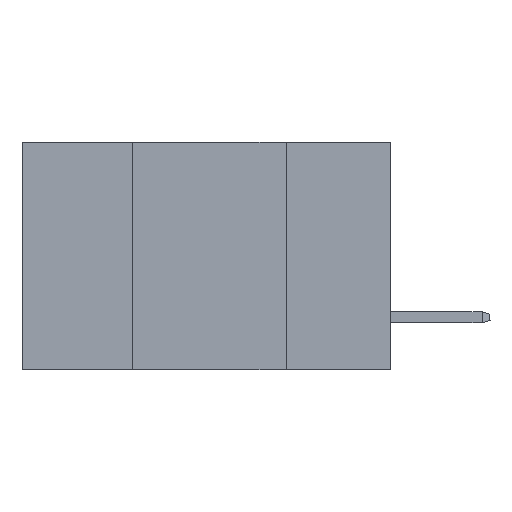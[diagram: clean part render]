
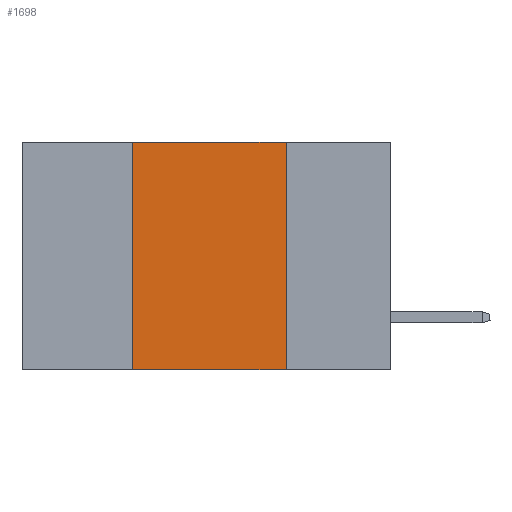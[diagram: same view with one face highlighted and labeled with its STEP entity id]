
A CAD part, left-side view. The second image highlights one B-rep face of the part: STEP entity #1698.
In plain terms, the highlighted planar face has unit normal (-1, 0, 0).
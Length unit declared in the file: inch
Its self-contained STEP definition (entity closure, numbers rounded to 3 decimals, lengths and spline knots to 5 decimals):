
#1095 = EDGE_CURVE ( 'NONE', #9346, #10973, #15724, .T. ) ;
#1698 = ADVANCED_FACE ( 'NONE', ( #9740 ), #7026, .F. ) ;
#1871 = DIRECTION ( 'NONE',  ( 1., 0., 0. ) ) ;
#2269 = DIRECTION ( 'NONE',  ( 0., -1., 0. ) ) ;
#2496 = ORIENTED_EDGE ( 'NONE', *, *, #2979, .F. ) ;
#2635 = EDGE_CURVE ( 'NONE', #7552, #4142, #11220, .T. ) ;
#2979 = EDGE_CURVE ( 'NONE', #9346, #7552, #15847, .T. ) ;
#3307 = CARTESIAN_POINT ( 'NONE',  ( 0., 0.17, 0. ) ) ;
#4142 = VERTEX_POINT ( 'NONE', #6917 ) ;
#4414 = CARTESIAN_POINT ( 'NONE',  ( 0., 0.42, 0. ) ) ;
#5377 = CARTESIAN_POINT ( 'NONE',  ( 0., 0.6, 0. ) ) ;
#5730 = CARTESIAN_POINT ( 'NONE',  ( 0., 0.42, -0.37 ) ) ;
#5921 = VECTOR ( 'NONE', #2269, 39.37008 ) ;
#6225 = LINE ( 'NONE', #3307, #9540 ) ;
#6917 = CARTESIAN_POINT ( 'NONE',  ( 0., 0.17, 0. ) ) ;
#6982 = AXIS2_PLACEMENT_3D ( 'NONE', #5377, #1871, #15802 ) ;
#7026 = PLANE ( 'NONE',  #6982 ) ;
#7552 = VERTEX_POINT ( 'NONE', #11511 ) ;
#8366 = VECTOR ( 'NONE', #16881, 39.37008 ) ;
#8958 = ORIENTED_EDGE ( 'NONE', *, *, #2635, .F. ) ;
#9346 = VERTEX_POINT ( 'NONE', #5730 ) ;
#9540 = VECTOR ( 'NONE', #10440, 39.37008 ) ;
#9740 = FACE_OUTER_BOUND ( 'NONE', #14753, .T. ) ;
#10440 = DIRECTION ( 'NONE',  ( 0., 0., -1. ) ) ;
#10973 = VERTEX_POINT ( 'NONE', #17334 ) ;
#11220 = LINE ( 'NONE', #16680, #5921 ) ;
#11511 = CARTESIAN_POINT ( 'NONE',  ( 0., 0.42, 0. ) ) ;
#11795 = DIRECTION ( 'NONE',  ( 0., -1., 0. ) ) ;
#12892 = VECTOR ( 'NONE', #11795, 39.37008 ) ;
#13136 = EDGE_CURVE ( 'NONE', #4142, #10973, #6225, .T. ) ;
#14753 = EDGE_LOOP ( 'NONE', ( #17250, #8958, #2496, #18028 ) ) ;
#15724 = LINE ( 'NONE', #16200, #12892 ) ;
#15802 = DIRECTION ( 'NONE',  ( 0., 0., -1. ) ) ;
#15847 = LINE ( 'NONE', #4414, #8366 ) ;
#16200 = CARTESIAN_POINT ( 'NONE',  ( 0., 0.6, -0.37 ) ) ;
#16680 = CARTESIAN_POINT ( 'NONE',  ( 0., 0.6, 0. ) ) ;
#16881 = DIRECTION ( 'NONE',  ( 0., 0., 1. ) ) ;
#17250 = ORIENTED_EDGE ( 'NONE', *, *, #13136, .F. ) ;
#17334 = CARTESIAN_POINT ( 'NONE',  ( 0., 0.17, -0.37 ) ) ;
#18028 = ORIENTED_EDGE ( 'NONE', *, *, #1095, .T. ) ;
